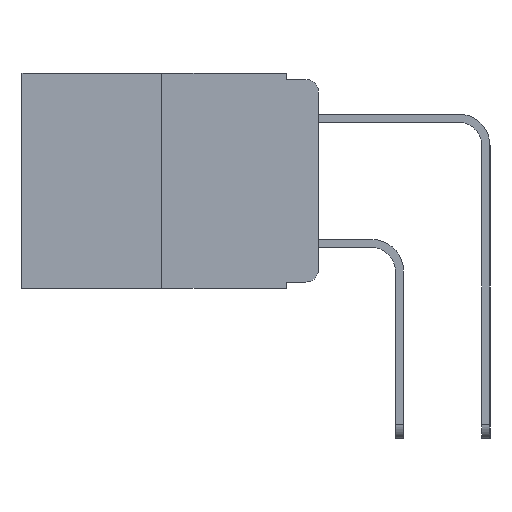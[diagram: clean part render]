
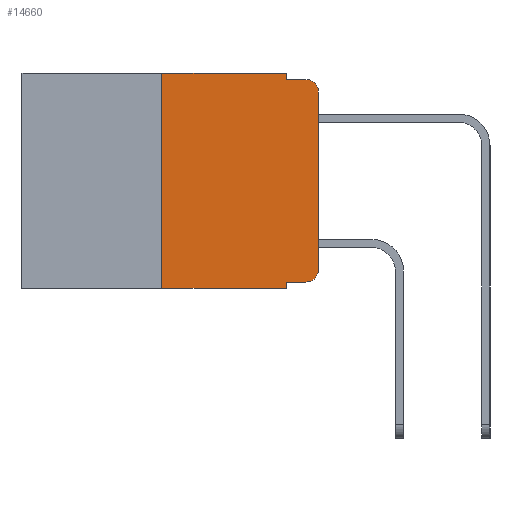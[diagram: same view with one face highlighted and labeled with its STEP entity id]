
A CAD part, left-side view. The second image highlights one B-rep face of the part: STEP entity #14660.
In plain terms, the highlighted planar face has unit normal (-1, 0, 0).
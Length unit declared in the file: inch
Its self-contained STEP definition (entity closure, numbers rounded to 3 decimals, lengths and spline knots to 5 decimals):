
#48 = CARTESIAN_POINT ( 'NONE',  ( 0., 0., 0. ) ) ;
#470 = VERTEX_POINT ( 'NONE', #1571 ) ;
#616 = AXIS2_PLACEMENT_3D ( 'NONE', #2983, #13461, #4493 ) ;
#650 = DIRECTION ( 'NONE',  ( 0., -1., 0. ) ) ;
#1520 = VERTEX_POINT ( 'NONE', #12808 ) ;
#1571 = CARTESIAN_POINT ( 'NONE',  ( 0., 0.051, 0. ) ) ;
#1621 = EDGE_CURVE ( 'NONE', #13741, #8699, #6679, .T. ) ;
#1749 = ORIENTED_EDGE ( 'NONE', *, *, #11593, .T. ) ;
#1866 = DIRECTION ( 'NONE',  ( -1., 0., 0. ) ) ;
#1884 = ORIENTED_EDGE ( 'NONE', *, *, #10569, .T. ) ;
#1904 = ORIENTED_EDGE ( 'NONE', *, *, #6629, .F. ) ;
#2160 = ORIENTED_EDGE ( 'NONE', *, *, #5591, .F. ) ;
#2363 = AXIS2_PLACEMENT_3D ( 'NONE', #2722, #7314, #11887 ) ;
#2498 = ORIENTED_EDGE ( 'NONE', *, *, #4715, .F. ) ;
#2586 = EDGE_CURVE ( 'NONE', #13741, #7488, #5449, .T. ) ;
#2603 = CARTESIAN_POINT ( 'NONE',  ( 0., 0.02, -0.333 ) ) ;
#2653 = EDGE_LOOP ( 'NONE', ( #1749, #1884, #1904, #2160, #2498, #2911, #3061, #3155, #3533, #3572 ) ) ;
#2722 = CARTESIAN_POINT ( 'NONE',  ( 0., 0.473, 0. ) ) ;
#2774 = LINE ( 'NONE', #15098, #17850 ) ;
#2908 = CARTESIAN_POINT ( 'NONE',  ( 0., 0.051, -0.333 ) ) ;
#2911 = ORIENTED_EDGE ( 'NONE', *, *, #3585, .F. ) ;
#2983 = CARTESIAN_POINT ( 'NONE',  ( 0., 0.02, -0.03 ) ) ;
#3061 = ORIENTED_EDGE ( 'NONE', *, *, #8884, .T. ) ;
#3155 = ORIENTED_EDGE ( 'NONE', *, *, #2586, .F. ) ;
#3184 = LINE ( 'NONE', #5870, #10197 ) ;
#3296 = VECTOR ( 'NONE', #8747, 39.37008 ) ;
#3533 = ORIENTED_EDGE ( 'NONE', *, *, #1621, .T. ) ;
#3572 = ORIENTED_EDGE ( 'NONE', *, *, #4602, .T. ) ;
#3585 = EDGE_CURVE ( 'NONE', #11715, #15863, #6861, .T. ) ;
#3731 = CIRCLE ( 'NONE', #3819, 0.02 ) ;
#3819 = AXIS2_PLACEMENT_3D ( 'NONE', #10797, #1866, #12321 ) ;
#4247 = DIRECTION ( 'NONE',  ( 0., 0., -1. ) ) ;
#4382 = VERTEX_POINT ( 'NONE', #15877 ) ;
#4493 = DIRECTION ( 'NONE',  ( 0., 0., -1. ) ) ;
#4602 = EDGE_CURVE ( 'NONE', #8699, #4382, #3731, .T. ) ;
#4618 = CARTESIAN_POINT ( 'NONE',  ( 0., 0., -0.03 ) ) ;
#4715 = EDGE_CURVE ( 'NONE', #15863, #470, #13325, .T. ) ;
#5069 = VECTOR ( 'NONE', #13585, 39.37008 ) ;
#5217 = DIRECTION ( 'NONE',  ( 0., -1., 0. ) ) ;
#5449 = LINE ( 'NONE', #14625, #12470 ) ;
#5591 = EDGE_CURVE ( 'NONE', #470, #1520, #2774, .T. ) ;
#5870 = CARTESIAN_POINT ( 'NONE',  ( 0., 0.473, -0.343 ) ) ;
#6618 = VERTEX_POINT ( 'NONE', #4618 ) ;
#6629 = EDGE_CURVE ( 'NONE', #1520, #15215, #9065, .T. ) ;
#6679 = LINE ( 'NONE', #2908, #9701 ) ;
#6861 = LINE ( 'NONE', #12971, #3296 ) ;
#7314 = DIRECTION ( 'NONE',  ( 1., 0., 0. ) ) ;
#7445 = DIRECTION ( 'NONE',  ( 0., -1., 0. ) ) ;
#7488 = VERTEX_POINT ( 'NONE', #16643 ) ;
#7679 = DIRECTION ( 'NONE',  ( 0., 0., 1. ) ) ;
#7718 = CARTESIAN_POINT ( 'NONE',  ( 0., 0.051, -0.01 ) ) ;
#8091 = LINE ( 'NONE', #48, #11520 ) ;
#8699 = VERTEX_POINT ( 'NONE', #2603 ) ;
#8747 = DIRECTION ( 'NONE',  ( 0., 0., 1. ) ) ;
#8820 = CARTESIAN_POINT ( 'NONE',  ( 0., 0.051, -0.333 ) ) ;
#8884 = EDGE_CURVE ( 'NONE', #11715, #7488, #3184, .T. ) ;
#9065 = LINE ( 'NONE', #7718, #5069 ) ;
#9701 = VECTOR ( 'NONE', #5217, 39.37008 ) ;
#10197 = VECTOR ( 'NONE', #7445, 39.37008 ) ;
#10569 = EDGE_CURVE ( 'NONE', #6618, #15215, #14352, .T. ) ;
#10797 = CARTESIAN_POINT ( 'NONE',  ( 0., 0.02, -0.313 ) ) ;
#11131 = CARTESIAN_POINT ( 'NONE',  ( 0., 0.473, 0. ) ) ;
#11294 = PLANE ( 'NONE',  #2363 ) ;
#11360 = CARTESIAN_POINT ( 'NONE',  ( 0., 0.02, -0.01 ) ) ;
#11520 = VECTOR ( 'NONE', #7679, 39.37008 ) ;
#11593 = EDGE_CURVE ( 'NONE', #4382, #6618, #8091, .T. ) ;
#11715 = VERTEX_POINT ( 'NONE', #16704 ) ;
#11887 = DIRECTION ( 'NONE',  ( 0., 0., -1. ) ) ;
#12278 = DIRECTION ( 'NONE',  ( 0., 0., -1. ) ) ;
#12321 = DIRECTION ( 'NONE',  ( 0., 0., -1. ) ) ;
#12470 = VECTOR ( 'NONE', #4247, 39.37008 ) ;
#12808 = CARTESIAN_POINT ( 'NONE',  ( 0., 0.051, -0.01 ) ) ;
#12971 = CARTESIAN_POINT ( 'NONE',  ( 0., 0.25, 0. ) ) ;
#13325 = LINE ( 'NONE', #11131, #16596 ) ;
#13332 = FACE_OUTER_BOUND ( 'NONE', #2653, .T. ) ;
#13461 = DIRECTION ( 'NONE',  ( -1., 0., 0. ) ) ;
#13585 = DIRECTION ( 'NONE',  ( 0., -1., 0. ) ) ;
#13741 = VERTEX_POINT ( 'NONE', #8820 ) ;
#14352 = CIRCLE ( 'NONE', #616, 0.02 ) ;
#14625 = CARTESIAN_POINT ( 'NONE',  ( 0., 0.051, 0. ) ) ;
#14660 = ADVANCED_FACE ( 'NONE', ( #13332 ), #11294, .F. ) ;
#15098 = CARTESIAN_POINT ( 'NONE',  ( 0., 0.051, 0. ) ) ;
#15215 = VERTEX_POINT ( 'NONE', #11360 ) ;
#15863 = VERTEX_POINT ( 'NONE', #17123 ) ;
#15877 = CARTESIAN_POINT ( 'NONE',  ( 0., 0., -0.313 ) ) ;
#16596 = VECTOR ( 'NONE', #650, 39.37008 ) ;
#16643 = CARTESIAN_POINT ( 'NONE',  ( 0., 0.051, -0.343 ) ) ;
#16704 = CARTESIAN_POINT ( 'NONE',  ( 0., 0.25, -0.343 ) ) ;
#17123 = CARTESIAN_POINT ( 'NONE',  ( 0., 0.25, 0. ) ) ;
#17850 = VECTOR ( 'NONE', #12278, 39.37008 ) ;
